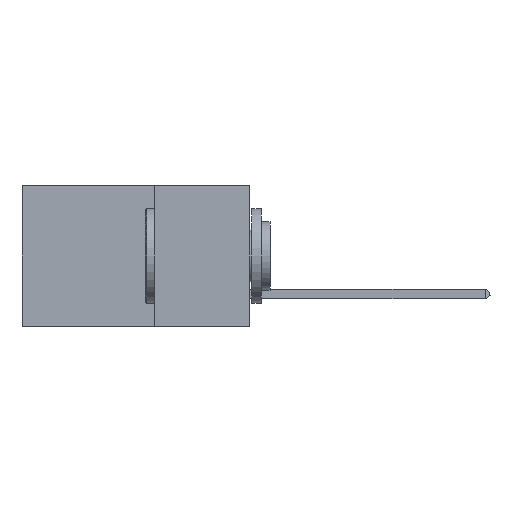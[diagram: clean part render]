
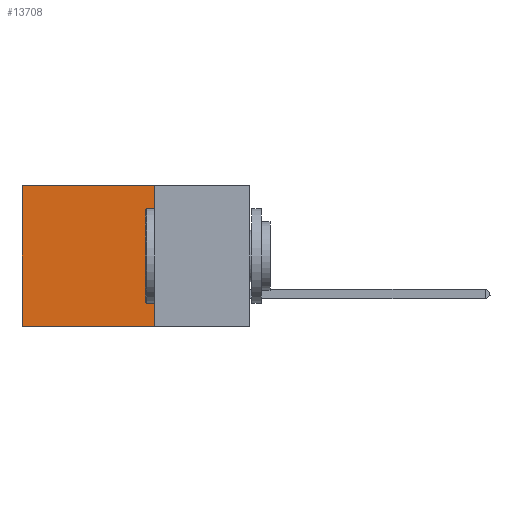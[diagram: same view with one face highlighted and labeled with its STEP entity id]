
A CAD part, left-side view. The second image highlights one B-rep face of the part: STEP entity #13708.
In plain terms, the highlighted planar face has unit normal (-1, 0, 0).
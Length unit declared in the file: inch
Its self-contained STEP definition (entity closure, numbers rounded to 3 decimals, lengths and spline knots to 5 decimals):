
#75 = FACE_OUTER_BOUND ( 'NONE', #7906, .T. ) ;
#310 = LINE ( 'NONE', #4952, #3909 ) ;
#653 = CARTESIAN_POINT ( 'NONE',  ( 0.2875, 0.6, -0.37 ) ) ;
#1030 = EDGE_CURVE ( 'NONE', #4153, #4114, #8868, .T. ) ;
#1854 = VERTEX_POINT ( 'NONE', #653 ) ;
#1989 = CARTESIAN_POINT ( 'NONE',  ( 0.2875, 0.25, 0. ) ) ;
#2175 = EDGE_CURVE ( 'NONE', #4153, #13446, #15521, .T. ) ;
#2738 = CARTESIAN_POINT ( 'NONE',  ( 0.2875, 0.25, -0.37 ) ) ;
#3020 = DIRECTION ( 'NONE',  ( 0., 1., 0. ) ) ;
#3909 = VECTOR ( 'NONE', #5113, 39.37008 ) ;
#3981 = DIRECTION ( 'NONE',  ( 0., 1., 0. ) ) ;
#4114 = VERTEX_POINT ( 'NONE', #6685 ) ;
#4153 = VERTEX_POINT ( 'NONE', #1989 ) ;
#4662 = VECTOR ( 'NONE', #3020, 39.37008 ) ;
#4838 = DIRECTION ( 'NONE',  ( 0., 0., -1. ) ) ;
#4952 = CARTESIAN_POINT ( 'NONE',  ( 0.2875, 0.6, 0. ) ) ;
#5113 = DIRECTION ( 'NONE',  ( 0., 0., -1. ) ) ;
#5205 = ORIENTED_EDGE ( 'NONE', *, *, #12936, .F. ) ;
#6279 = DIRECTION ( 'NONE',  ( 0., 0., -1. ) ) ;
#6685 = CARTESIAN_POINT ( 'NONE',  ( 0.2875, 0.6, 0. ) ) ;
#6703 = VECTOR ( 'NONE', #3981, 39.37008 ) ;
#7674 = CARTESIAN_POINT ( 'NONE',  ( 0.2875, 0.25, 0. ) ) ;
#7906 = EDGE_LOOP ( 'NONE', ( #11980, #5205, #7991, #14127 ) ) ;
#7991 = ORIENTED_EDGE ( 'NONE', *, *, #2175, .F. ) ;
#8249 = AXIS2_PLACEMENT_3D ( 'NONE', #15027, #13634, #6279 ) ;
#8868 = LINE ( 'NONE', #7674, #6703 ) ;
#9131 = CARTESIAN_POINT ( 'NONE',  ( 0.2875, 0.25, -0.37 ) ) ;
#9316 = LINE ( 'NONE', #9131, #4662 ) ;
#10880 = CARTESIAN_POINT ( 'NONE',  ( 0.2875, 0.25, 0. ) ) ;
#11980 = ORIENTED_EDGE ( 'NONE', *, *, #16195, .T. ) ;
#12798 = VECTOR ( 'NONE', #4838, 39.37008 ) ;
#12936 = EDGE_CURVE ( 'NONE', #13446, #1854, #9316, .T. ) ;
#13446 = VERTEX_POINT ( 'NONE', #2738 ) ;
#13634 = DIRECTION ( 'NONE',  ( 1., 0., 0. ) ) ;
#13708 = ADVANCED_FACE ( 'NONE', ( #75 ), #13794, .F. ) ;
#13794 = PLANE ( 'NONE',  #8249 ) ;
#14127 = ORIENTED_EDGE ( 'NONE', *, *, #1030, .T. ) ;
#15027 = CARTESIAN_POINT ( 'NONE',  ( 0.2875, 0.25, 0. ) ) ;
#15521 = LINE ( 'NONE', #10880, #12798 ) ;
#16195 = EDGE_CURVE ( 'NONE', #4114, #1854, #310, .T. ) ;
